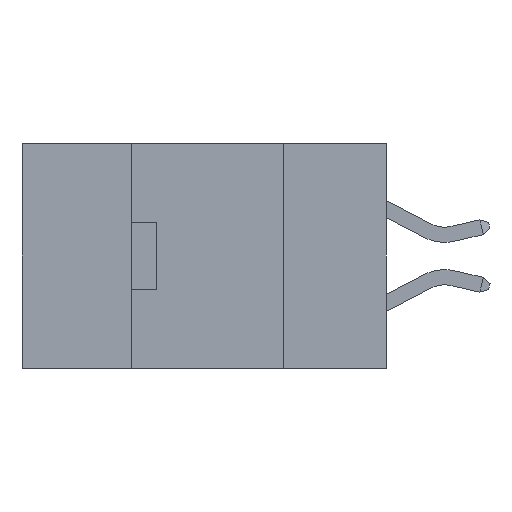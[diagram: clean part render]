
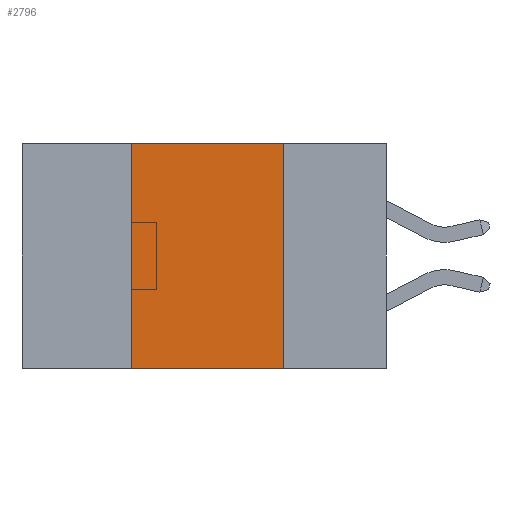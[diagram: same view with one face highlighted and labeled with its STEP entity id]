
A CAD part, left-side view. The second image highlights one B-rep face of the part: STEP entity #2796.
In plain terms, the highlighted planar face has unit normal (-1, 0, 0).
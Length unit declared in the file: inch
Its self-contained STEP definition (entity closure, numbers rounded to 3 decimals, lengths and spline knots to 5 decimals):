
#1003 = CARTESIAN_POINT ( 'NONE',  ( 0., 0.42, -0.37 ) ) ;
#1331 = EDGE_CURVE ( 'NONE', #11259, #23700, #20273, .T. ) ;
#1426 = PLANE ( 'NONE',  #16120 ) ;
#1802 = CARTESIAN_POINT ( 'NONE',  ( 0., 0.42, 0. ) ) ;
#2101 = VECTOR ( 'NONE', #14590, 39.37008 ) ;
#2530 = CARTESIAN_POINT ( 'NONE',  ( 0., 0.17, -0.37 ) ) ;
#2796 = ADVANCED_FACE ( 'NONE', ( #14989 ), #1426, .F. ) ;
#3508 = DIRECTION ( 'NONE',  ( 1., 0., 0. ) ) ;
#4202 = EDGE_LOOP ( 'NONE', ( #24265, #10000, #25690, #6022 ) ) ;
#6022 = ORIENTED_EDGE ( 'NONE', *, *, #14239, .T. ) ;
#6869 = VERTEX_POINT ( 'NONE', #1003 ) ;
#6907 = CARTESIAN_POINT ( 'NONE',  ( 0., 0.6, -0.37 ) ) ;
#7081 = VECTOR ( 'NONE', #23400, 39.37008 ) ;
#7591 = LINE ( 'NONE', #20832, #2101 ) ;
#7737 = LINE ( 'NONE', #6907, #7081 ) ;
#8463 = CARTESIAN_POINT ( 'NONE',  ( 0., 0.42, -0.37 ) ) ;
#10000 = ORIENTED_EDGE ( 'NONE', *, *, #22899, .F. ) ;
#10001 = VECTOR ( 'NONE', #10509, 39.37008 ) ;
#10509 = DIRECTION ( 'NONE',  ( 0., 0., 1. ) ) ;
#11259 = VERTEX_POINT ( 'NONE', #21296 ) ;
#13516 = EDGE_CURVE ( 'NONE', #6869, #19595, #25873, .T. ) ;
#14239 = EDGE_CURVE ( 'NONE', #6869, #23700, #7737, .T. ) ;
#14590 = DIRECTION ( 'NONE',  ( 0., -1., 0. ) ) ;
#14989 = FACE_OUTER_BOUND ( 'NONE', #4202, .T. ) ;
#16120 = AXIS2_PLACEMENT_3D ( 'NONE', #21982, #3508, #17888 ) ;
#17888 = DIRECTION ( 'NONE',  ( 0., 0., -1. ) ) ;
#19592 = VECTOR ( 'NONE', #19835, 39.37008 ) ;
#19595 = VERTEX_POINT ( 'NONE', #1802 ) ;
#19835 = DIRECTION ( 'NONE',  ( 0., 0., -1. ) ) ;
#20273 = LINE ( 'NONE', #23923, #19592 ) ;
#20832 = CARTESIAN_POINT ( 'NONE',  ( 0., 0.6, 0. ) ) ;
#21296 = CARTESIAN_POINT ( 'NONE',  ( 0., 0.17, 0. ) ) ;
#21982 = CARTESIAN_POINT ( 'NONE',  ( 0., 0.6, 0. ) ) ;
#22899 = EDGE_CURVE ( 'NONE', #19595, #11259, #7591, .T. ) ;
#23400 = DIRECTION ( 'NONE',  ( 0., -1., 0. ) ) ;
#23700 = VERTEX_POINT ( 'NONE', #2530 ) ;
#23923 = CARTESIAN_POINT ( 'NONE',  ( 0., 0.17, -0.37 ) ) ;
#24265 = ORIENTED_EDGE ( 'NONE', *, *, #1331, .F. ) ;
#25690 = ORIENTED_EDGE ( 'NONE', *, *, #13516, .F. ) ;
#25873 = LINE ( 'NONE', #8463, #10001 ) ;
